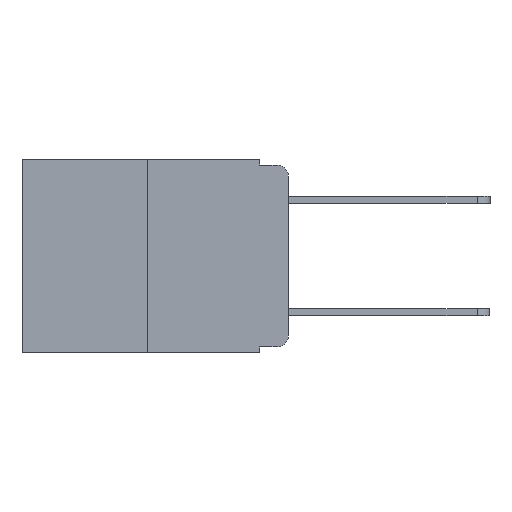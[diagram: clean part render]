
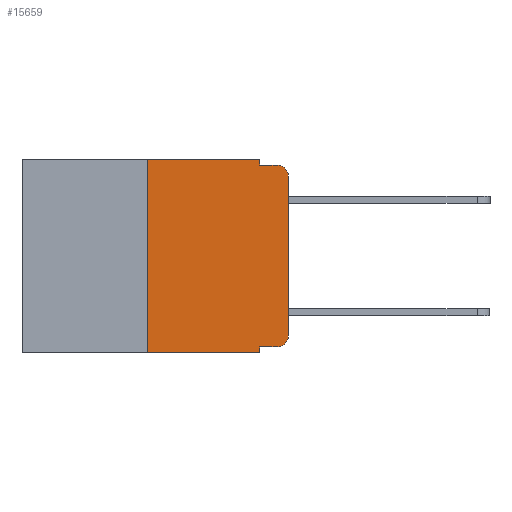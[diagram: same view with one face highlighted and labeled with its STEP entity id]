
A CAD part, left-side view. The second image highlights one B-rep face of the part: STEP entity #15659.
In plain terms, the highlighted planar face has unit normal (-1, 0, 0).
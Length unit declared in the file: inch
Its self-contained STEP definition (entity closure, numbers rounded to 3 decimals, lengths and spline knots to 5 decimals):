
#127 = DIRECTION ( 'NONE',  ( 0., 0., 1. ) ) ;
#363 = DIRECTION ( 'NONE',  ( -1., 0., 0. ) ) ;
#694 = CARTESIAN_POINT ( 'NONE',  ( 0., 0.02, -0.01 ) ) ;
#742 = VERTEX_POINT ( 'NONE', #20940 ) ;
#763 = EDGE_LOOP ( 'NONE', ( #10866, #3258, #5696, #5075, #7916, #3735, #10994, #7053, #13741, #1650 ) ) ;
#1341 = CARTESIAN_POINT ( 'NONE',  ( 0., 0.02, -0.03 ) ) ;
#1557 = VECTOR ( 'NONE', #10306, 39.37008 ) ;
#1628 = AXIS2_PLACEMENT_3D ( 'NONE', #16103, #8380, #21739 ) ;
#1650 = ORIENTED_EDGE ( 'NONE', *, *, #22470, .T. ) ;
#1678 = VERTEX_POINT ( 'NONE', #4793 ) ;
#1758 = CARTESIAN_POINT ( 'NONE',  ( 0., 0.051, 0. ) ) ;
#1831 = EDGE_CURVE ( 'NONE', #3477, #12152, #12779, .T. ) ;
#2133 = AXIS2_PLACEMENT_3D ( 'NONE', #12348, #363, #14261 ) ;
#2138 = CARTESIAN_POINT ( 'NONE',  ( 0., 0.051, -0.333 ) ) ;
#2555 = DIRECTION ( 'NONE',  ( 0., -1., 0. ) ) ;
#2926 = AXIS2_PLACEMENT_3D ( 'NONE', #1341, #15167, #3367 ) ;
#3258 = ORIENTED_EDGE ( 'NONE', *, *, #20389, .T. ) ;
#3367 = DIRECTION ( 'NONE',  ( 0., 0., -1. ) ) ;
#3477 = VERTEX_POINT ( 'NONE', #19187 ) ;
#3735 = ORIENTED_EDGE ( 'NONE', *, *, #13271, .F. ) ;
#4793 = CARTESIAN_POINT ( 'NONE',  ( 0., 0.02, -0.333 ) ) ;
#5075 = ORIENTED_EDGE ( 'NONE', *, *, #15233, .F. ) ;
#5133 = VECTOR ( 'NONE', #8808, 39.37008 ) ;
#5402 = VERTEX_POINT ( 'NONE', #694 ) ;
#5696 = ORIENTED_EDGE ( 'NONE', *, *, #22440, .F. ) ;
#6403 = LINE ( 'NONE', #1758, #21148 ) ;
#6536 = CARTESIAN_POINT ( 'NONE',  ( 0., 0.051, -0.333 ) ) ;
#6558 = LINE ( 'NONE', #14889, #15743 ) ;
#7053 = ORIENTED_EDGE ( 'NONE', *, *, #12301, .F. ) ;
#7522 = VECTOR ( 'NONE', #7849, 39.37008 ) ;
#7822 = CARTESIAN_POINT ( 'NONE',  ( 0., 0., -0.03 ) ) ;
#7849 = DIRECTION ( 'NONE',  ( 0., -1., 0. ) ) ;
#7916 = ORIENTED_EDGE ( 'NONE', *, *, #1831, .F. ) ;
#7918 = EDGE_CURVE ( 'NONE', #19847, #742, #24464, .T. ) ;
#8122 = EDGE_CURVE ( 'NONE', #23039, #1678, #10329, .T. ) ;
#8380 = DIRECTION ( 'NONE',  ( 1., 0., 0. ) ) ;
#8569 = CIRCLE ( 'NONE', #2926, 0.02 ) ;
#8735 = CARTESIAN_POINT ( 'NONE',  ( 0., 0.473, 0. ) ) ;
#8808 = DIRECTION ( 'NONE',  ( 0., 0., 1. ) ) ;
#9231 = VERTEX_POINT ( 'NONE', #7822 ) ;
#9877 = EDGE_CURVE ( 'NONE', #20697, #9231, #12979, .T. ) ;
#10020 = VECTOR ( 'NONE', #19362, 39.37008 ) ;
#10306 = DIRECTION ( 'NONE',  ( 0., -1., 0. ) ) ;
#10329 = LINE ( 'NONE', #6536, #14838 ) ;
#10458 = LINE ( 'NONE', #12670, #5133 ) ;
#10866 = ORIENTED_EDGE ( 'NONE', *, *, #9877, .T. ) ;
#10978 = CARTESIAN_POINT ( 'NONE',  ( 0., 0.051, -0.01 ) ) ;
#10994 = ORIENTED_EDGE ( 'NONE', *, *, #7918, .T. ) ;
#11267 = CARTESIAN_POINT ( 'NONE',  ( 0., 0.051, 0. ) ) ;
#12138 = CARTESIAN_POINT ( 'NONE',  ( 0., 0., 0. ) ) ;
#12152 = VERTEX_POINT ( 'NONE', #11267 ) ;
#12179 = CIRCLE ( 'NONE', #2133, 0.02 ) ;
#12301 = EDGE_CURVE ( 'NONE', #23039, #742, #6403, .T. ) ;
#12348 = CARTESIAN_POINT ( 'NONE',  ( 0., 0.02, -0.313 ) ) ;
#12670 = CARTESIAN_POINT ( 'NONE',  ( 0., 0.25, 0. ) ) ;
#12779 = LINE ( 'NONE', #8735, #7522 ) ;
#12979 = LINE ( 'NONE', #12138, #17405 ) ;
#13271 = EDGE_CURVE ( 'NONE', #19847, #3477, #10458, .T. ) ;
#13741 = ORIENTED_EDGE ( 'NONE', *, *, #8122, .T. ) ;
#14005 = VERTEX_POINT ( 'NONE', #10978 ) ;
#14261 = DIRECTION ( 'NONE',  ( 0., 0., -1. ) ) ;
#14838 = VECTOR ( 'NONE', #2555, 39.37008 ) ;
#14889 = CARTESIAN_POINT ( 'NONE',  ( 0., 0.051, 0. ) ) ;
#15167 = DIRECTION ( 'NONE',  ( -1., 0., 0. ) ) ;
#15233 = EDGE_CURVE ( 'NONE', #12152, #14005, #6558, .T. ) ;
#15659 = ADVANCED_FACE ( 'NONE', ( #20096 ), #19852, .F. ) ;
#15743 = VECTOR ( 'NONE', #18631, 39.37008 ) ;
#16103 = CARTESIAN_POINT ( 'NONE',  ( 0., 0.473, 0. ) ) ;
#17405 = VECTOR ( 'NONE', #127, 39.37008 ) ;
#17408 = DIRECTION ( 'NONE',  ( 0., 0., -1. ) ) ;
#18631 = DIRECTION ( 'NONE',  ( 0., 0., -1. ) ) ;
#19187 = CARTESIAN_POINT ( 'NONE',  ( 0., 0.25, 0. ) ) ;
#19362 = DIRECTION ( 'NONE',  ( 0., -1., 0. ) ) ;
#19745 = CARTESIAN_POINT ( 'NONE',  ( 0., 0.051, -0.01 ) ) ;
#19847 = VERTEX_POINT ( 'NONE', #24467 ) ;
#19852 = PLANE ( 'NONE',  #1628 ) ;
#20096 = FACE_OUTER_BOUND ( 'NONE', #763, .T. ) ;
#20389 = EDGE_CURVE ( 'NONE', #9231, #5402, #8569, .T. ) ;
#20697 = VERTEX_POINT ( 'NONE', #23497 ) ;
#20940 = CARTESIAN_POINT ( 'NONE',  ( 0., 0.051, -0.343 ) ) ;
#21148 = VECTOR ( 'NONE', #17408, 39.37008 ) ;
#21343 = CARTESIAN_POINT ( 'NONE',  ( 0., 0.473, -0.343 ) ) ;
#21739 = DIRECTION ( 'NONE',  ( 0., 0., -1. ) ) ;
#22165 = LINE ( 'NONE', #19745, #1557 ) ;
#22440 = EDGE_CURVE ( 'NONE', #14005, #5402, #22165, .T. ) ;
#22470 = EDGE_CURVE ( 'NONE', #1678, #20697, #12179, .T. ) ;
#23039 = VERTEX_POINT ( 'NONE', #2138 ) ;
#23497 = CARTESIAN_POINT ( 'NONE',  ( 0., 0., -0.313 ) ) ;
#24464 = LINE ( 'NONE', #21343, #10020 ) ;
#24467 = CARTESIAN_POINT ( 'NONE',  ( 0., 0.25, -0.343 ) ) ;
